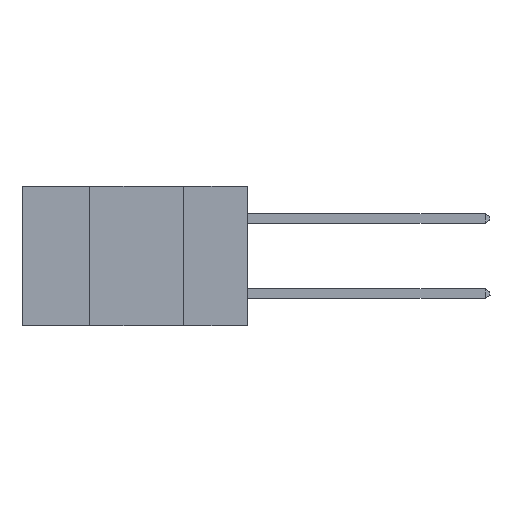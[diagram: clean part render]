
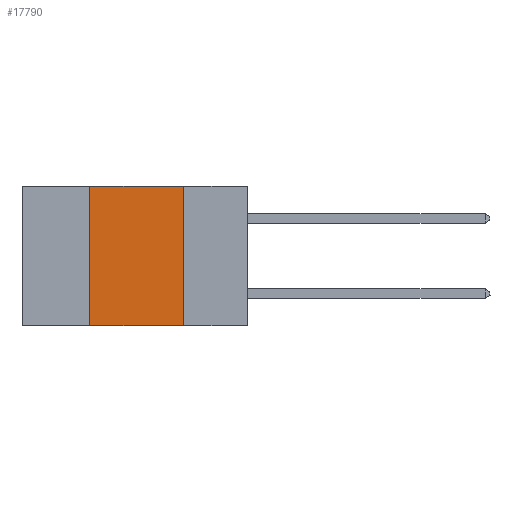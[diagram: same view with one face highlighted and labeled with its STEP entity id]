
A CAD part, left-side view. The second image highlights one B-rep face of the part: STEP entity #17790.
In plain terms, the highlighted planar face has unit normal (-1, 0, 0).
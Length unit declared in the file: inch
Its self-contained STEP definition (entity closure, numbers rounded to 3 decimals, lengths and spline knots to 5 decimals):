
#20 = CARTESIAN_POINT ( 'NONE',  ( 0., 0.42, -0.37 ) ) ;
#408 = LINE ( 'NONE', #18269, #9786 ) ;
#2026 = EDGE_CURVE ( 'NONE', #11758, #22742, #11164, .T. ) ;
#2339 = ORIENTED_EDGE ( 'NONE', *, *, #7173, .F. ) ;
#2743 = EDGE_CURVE ( 'NONE', #11758, #8636, #408, .T. ) ;
#4244 = VECTOR ( 'NONE', #21421, 39.37008 ) ;
#5893 = CARTESIAN_POINT ( 'NONE',  ( 0., 0.17, 0. ) ) ;
#6923 = FACE_OUTER_BOUND ( 'NONE', #10162, .T. ) ;
#7173 = EDGE_CURVE ( 'NONE', #17677, #8636, #21062, .T. ) ;
#7653 = DIRECTION ( 'NONE',  ( 0., -1., 0. ) ) ;
#8636 = VERTEX_POINT ( 'NONE', #21407 ) ;
#9360 = VECTOR ( 'NONE', #18299, 39.37008 ) ;
#9496 = CARTESIAN_POINT ( 'NONE',  ( 0., 0.6, 0. ) ) ;
#9727 = AXIS2_PLACEMENT_3D ( 'NONE', #9496, #18600, #15087 ) ;
#9786 = VECTOR ( 'NONE', #7653, 39.37008 ) ;
#10162 = EDGE_LOOP ( 'NONE', ( #2339, #16326, #21926, #13592 ) ) ;
#10886 = CARTESIAN_POINT ( 'NONE',  ( 0., 0.17, 0. ) ) ;
#11164 = LINE ( 'NONE', #16256, #4244 ) ;
#11758 = VERTEX_POINT ( 'NONE', #20 ) ;
#11983 = LINE ( 'NONE', #17159, #17551 ) ;
#12039 = CARTESIAN_POINT ( 'NONE',  ( 0., 0.42, 0. ) ) ;
#13219 = PLANE ( 'NONE',  #9727 ) ;
#13440 = DIRECTION ( 'NONE',  ( 0., -1., 0. ) ) ;
#13592 = ORIENTED_EDGE ( 'NONE', *, *, #2743, .T. ) ;
#15087 = DIRECTION ( 'NONE',  ( 0., 0., -1. ) ) ;
#16173 = EDGE_CURVE ( 'NONE', #22742, #17677, #11983, .T. ) ;
#16256 = CARTESIAN_POINT ( 'NONE',  ( 0., 0.42, 0. ) ) ;
#16326 = ORIENTED_EDGE ( 'NONE', *, *, #16173, .F. ) ;
#17159 = CARTESIAN_POINT ( 'NONE',  ( 0., 0.6, 0. ) ) ;
#17551 = VECTOR ( 'NONE', #13440, 39.37008 ) ;
#17677 = VERTEX_POINT ( 'NONE', #10886 ) ;
#17790 = ADVANCED_FACE ( 'NONE', ( #6923 ), #13219, .F. ) ;
#18269 = CARTESIAN_POINT ( 'NONE',  ( 0., 0.6, -0.37 ) ) ;
#18299 = DIRECTION ( 'NONE',  ( 0., 0., -1. ) ) ;
#18600 = DIRECTION ( 'NONE',  ( 1., 0., 0. ) ) ;
#21062 = LINE ( 'NONE', #5893, #9360 ) ;
#21407 = CARTESIAN_POINT ( 'NONE',  ( 0., 0.17, -0.37 ) ) ;
#21421 = DIRECTION ( 'NONE',  ( 0., 0., 1. ) ) ;
#21926 = ORIENTED_EDGE ( 'NONE', *, *, #2026, .F. ) ;
#22742 = VERTEX_POINT ( 'NONE', #12039 ) ;
